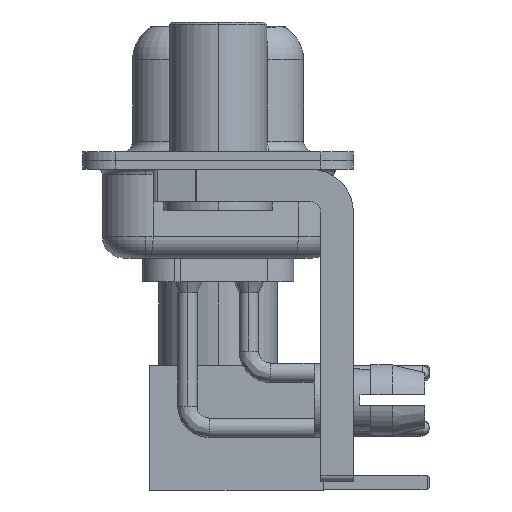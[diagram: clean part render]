
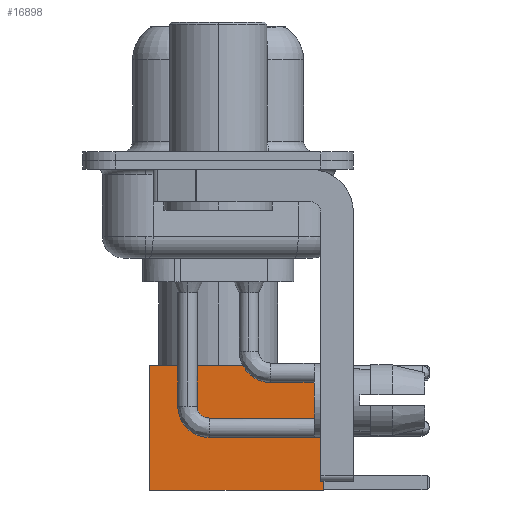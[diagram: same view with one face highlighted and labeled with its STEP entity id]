
A CAD part, left-side view. The second image highlights one B-rep face of the part: STEP entity #16898.
In plain terms, the highlighted face is planar.
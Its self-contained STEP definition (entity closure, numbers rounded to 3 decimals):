
#1242 = CARTESIAN_POINT ( 'NONE',  ( 2.875, 2.875, 8. ) ) ;
#3102 = ORIENTED_EDGE ( 'NONE', *, *, #14427, .F. ) ;
#4218 = DIRECTION ( 'NONE',  ( 0., 0., 1. ) ) ;
#5061 = EDGE_CURVE ( 'NONE', #18958, #9893, #20141, .T. ) ;
#7226 = LINE ( 'NONE', #23213, #23933 ) ;
#7466 = VECTOR ( 'NONE', #7839, 1000. ) ;
#7634 = ORIENTED_EDGE ( 'NONE', *, *, #5061, .T. ) ;
#7839 = DIRECTION ( 'NONE',  ( -1., 0., 0. ) ) ;
#8077 = DIRECTION ( 'NONE',  ( 0., 0., -1. ) ) ;
#8258 = ORIENTED_EDGE ( 'NONE', *, *, #15065, .T. ) ;
#8386 = AXIS2_PLACEMENT_3D ( 'NONE', #10516, #24671, #4218 ) ;
#9893 = VERTEX_POINT ( 'NONE', #13952 ) ;
#10516 = CARTESIAN_POINT ( 'NONE',  ( 2.875, 2.875, 0. ) ) ;
#10781 = PLANE ( 'NONE',  #8386 ) ;
#13037 = CARTESIAN_POINT ( 'NONE',  ( -2.875, 2.875, 8. ) ) ;
#13952 = CARTESIAN_POINT ( 'NONE',  ( 2.875, 2.875, 0. ) ) ;
#14104 = ORIENTED_EDGE ( 'NONE', *, *, #17156, .F. ) ;
#14395 = VERTEX_POINT ( 'NONE', #15517 ) ;
#14427 = EDGE_CURVE ( 'NONE', #18958, #20657, #15250, .T. ) ;
#14662 = VECTOR ( 'NONE', #17731, 1000. ) ;
#15065 = EDGE_CURVE ( 'NONE', #9893, #14395, #25930, .T. ) ;
#15250 = LINE ( 'NONE', #23219, #14662 ) ;
#15517 = CARTESIAN_POINT ( 'NONE',  ( -2.875, 2.875, 0. ) ) ;
#16898 = ADVANCED_FACE ( 'NONE', ( #18789 ), #10781, .T. ) ;
#17156 = EDGE_CURVE ( 'NONE', #20657, #14395, #7226, .T. ) ;
#17353 = VECTOR ( 'NONE', #8077, 1000. ) ;
#17599 = DIRECTION ( 'NONE',  ( 0., 0., -1. ) ) ;
#17731 = DIRECTION ( 'NONE',  ( -1., 0., 0. ) ) ;
#18789 = FACE_OUTER_BOUND ( 'NONE', #25234, .T. ) ;
#18958 = VERTEX_POINT ( 'NONE', #1242 ) ;
#20141 = LINE ( 'NONE', #25776, #17353 ) ;
#20657 = VERTEX_POINT ( 'NONE', #13037 ) ;
#23213 = CARTESIAN_POINT ( 'NONE',  ( -2.875, 2.875, 0. ) ) ;
#23219 = CARTESIAN_POINT ( 'NONE',  ( 0., 2.875, 8. ) ) ;
#23933 = VECTOR ( 'NONE', #17599, 1000. ) ;
#23959 = CARTESIAN_POINT ( 'NONE',  ( 0., 2.875, 0. ) ) ;
#24671 = DIRECTION ( 'NONE',  ( 0., 1., 0. ) ) ;
#25234 = EDGE_LOOP ( 'NONE', ( #7634, #8258, #14104, #3102 ) ) ;
#25776 = CARTESIAN_POINT ( 'NONE',  ( 2.875, 2.875, 0. ) ) ;
#25930 = LINE ( 'NONE', #23959, #7466 ) ;
